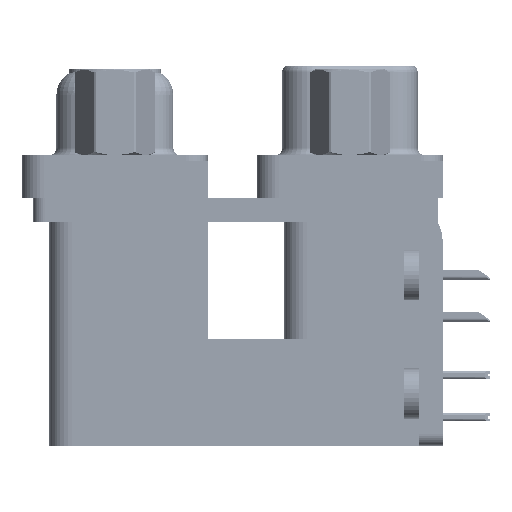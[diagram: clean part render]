
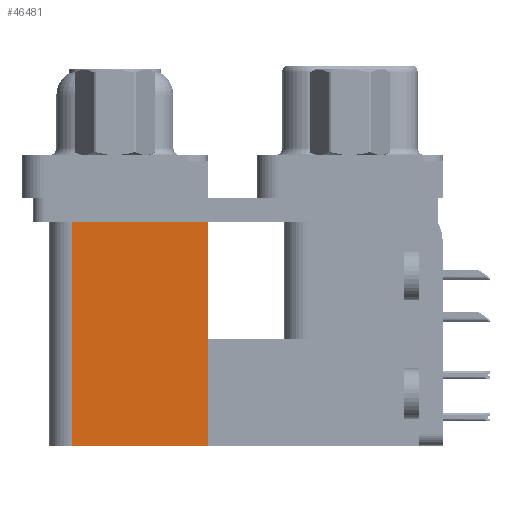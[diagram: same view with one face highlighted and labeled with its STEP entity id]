
A CAD part, left-side view. The second image highlights one B-rep face of the part: STEP entity #46481.
In plain terms, the highlighted planar face has unit normal (-1, 0, 0).
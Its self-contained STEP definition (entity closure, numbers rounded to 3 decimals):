
#3269 = CARTESIAN_POINT ( 'NONE',  ( 3.7, 9.6, -19.2 ) ) ;
#4367 = EDGE_CURVE ( 'NONE', #11130, #50641, #8300, .T. ) ;
#7995 = EDGE_LOOP ( 'NONE', ( #58819, #26884, #44513, #54481 ) ) ;
#8300 = LINE ( 'NONE', #3269, #26885 ) ;
#11130 = VERTEX_POINT ( 'NONE', #11514 ) ;
#11514 = CARTESIAN_POINT ( 'NONE',  ( 3.7, 9.6, -19.2 ) ) ;
#11684 = DIRECTION ( 'NONE',  ( 0., 0., 1. ) ) ;
#11871 = CARTESIAN_POINT ( 'NONE',  ( 3.7, 9.6, -19.2 ) ) ;
#15574 = CARTESIAN_POINT ( 'NONE',  ( 3.7, 9.6, -2.5 ) ) ;
#16278 = FACE_OUTER_BOUND ( 'NONE', #7995, .T. ) ;
#17035 = LINE ( 'NONE', #26782, #42175 ) ;
#17372 = EDGE_CURVE ( 'NONE', #11130, #59930, #61428, .T. ) ;
#20393 = PLANE ( 'NONE',  #37970 ) ;
#24738 = CARTESIAN_POINT ( 'NONE',  ( 3.7, 9.6, -2.5 ) ) ;
#25635 = LINE ( 'NONE', #15574, #39902 ) ;
#26782 = CARTESIAN_POINT ( 'NONE',  ( 3.7, 18.8, -19.2 ) ) ;
#26826 = CARTESIAN_POINT ( 'NONE',  ( 3.7, 18.8, -19.2 ) ) ;
#26884 = ORIENTED_EDGE ( 'NONE', *, *, #57401, .F. ) ;
#26885 = VECTOR ( 'NONE', #46677, 1000. ) ;
#29448 = DIRECTION ( 'NONE',  ( 0., 1., 0. ) ) ;
#29743 = VERTEX_POINT ( 'NONE', #34624 ) ;
#34542 = VECTOR ( 'NONE', #55454, 1000. ) ;
#34624 = CARTESIAN_POINT ( 'NONE',  ( 3.7, 18.8, -2.5 ) ) ;
#35176 = DIRECTION ( 'NONE',  ( 1., 0., 0. ) ) ;
#37970 = AXIS2_PLACEMENT_3D ( 'NONE', #11871, #35176, #39266 ) ;
#39266 = DIRECTION ( 'NONE',  ( 0., 0., -1. ) ) ;
#39902 = VECTOR ( 'NONE', #29448, 1000. ) ;
#42175 = VECTOR ( 'NONE', #11684, 1000. ) ;
#44513 = ORIENTED_EDGE ( 'NONE', *, *, #17372, .F. ) ;
#45579 = EDGE_CURVE ( 'NONE', #50641, #29743, #25635, .T. ) ;
#46481 = ADVANCED_FACE ( 'NONE', ( #16278 ), #20393, .F. ) ;
#46677 = DIRECTION ( 'NONE',  ( 0., 0., 1. ) ) ;
#50641 = VERTEX_POINT ( 'NONE', #24738 ) ;
#54481 = ORIENTED_EDGE ( 'NONE', *, *, #4367, .T. ) ;
#55454 = DIRECTION ( 'NONE',  ( 0., 1., 0. ) ) ;
#56697 = CARTESIAN_POINT ( 'NONE',  ( 3.7, 9.6, -19.2 ) ) ;
#57401 = EDGE_CURVE ( 'NONE', #59930, #29743, #17035, .T. ) ;
#58819 = ORIENTED_EDGE ( 'NONE', *, *, #45579, .T. ) ;
#59930 = VERTEX_POINT ( 'NONE', #26826 ) ;
#61428 = LINE ( 'NONE', #56697, #34542 ) ;
